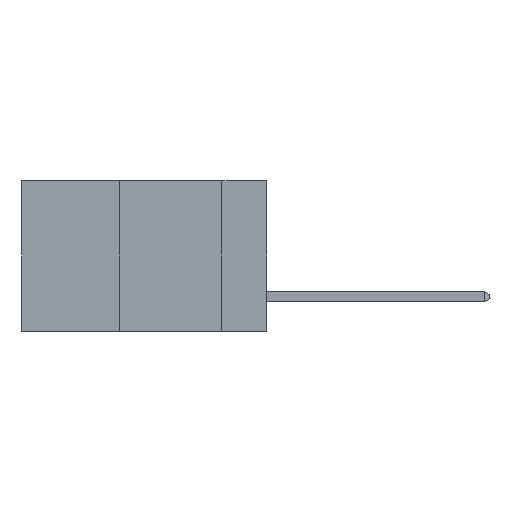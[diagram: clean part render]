
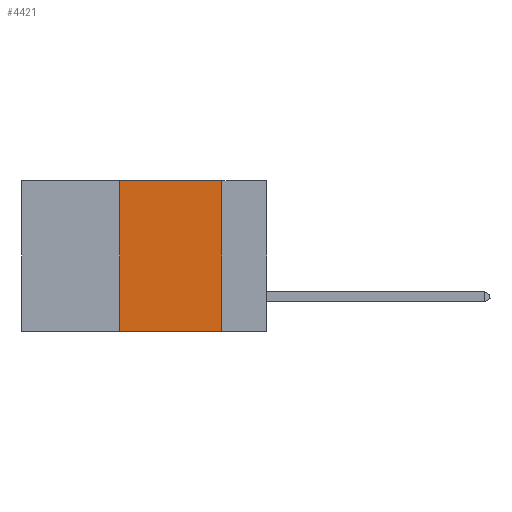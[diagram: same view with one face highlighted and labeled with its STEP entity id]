
A CAD part, left-side view. The second image highlights one B-rep face of the part: STEP entity #4421.
In plain terms, the highlighted planar face has unit normal (-1, 0, 0).
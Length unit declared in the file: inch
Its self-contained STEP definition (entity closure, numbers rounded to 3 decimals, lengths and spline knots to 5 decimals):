
#162 = DIRECTION ( 'NONE',  ( 1., 0., 0. ) ) ;
#515 = VECTOR ( 'NONE', #15361, 39.37008 ) ;
#859 = ORIENTED_EDGE ( 'NONE', *, *, #13508, .T. ) ;
#989 = FACE_OUTER_BOUND ( 'NONE', #6195, .T. ) ;
#1679 = CARTESIAN_POINT ( 'NONE',  ( 0., 0.6, -0.37 ) ) ;
#1713 = ORIENTED_EDGE ( 'NONE', *, *, #8844, .F. ) ;
#3783 = EDGE_CURVE ( 'NONE', #13636, #9212, #14231, .T. ) ;
#4421 = ADVANCED_FACE ( 'NONE', ( #989 ), #17350, .F. ) ;
#4846 = CARTESIAN_POINT ( 'NONE',  ( 0., 0.11, 0. ) ) ;
#4976 = LINE ( 'NONE', #8102, #515 ) ;
#6195 = EDGE_LOOP ( 'NONE', ( #6665, #7894, #1713, #859 ) ) ;
#6665 = ORIENTED_EDGE ( 'NONE', *, *, #19580, .F. ) ;
#7894 = ORIENTED_EDGE ( 'NONE', *, *, #3783, .F. ) ;
#8102 = CARTESIAN_POINT ( 'NONE',  ( 0., 0.36, 0. ) ) ;
#8215 = DIRECTION ( 'NONE',  ( 0., -1., 0. ) ) ;
#8844 = EDGE_CURVE ( 'NONE', #9439, #13636, #4976, .T. ) ;
#9212 = VERTEX_POINT ( 'NONE', #15399 ) ;
#9439 = VERTEX_POINT ( 'NONE', #16611 ) ;
#9733 = VECTOR ( 'NONE', #14005, 39.37008 ) ;
#12286 = CARTESIAN_POINT ( 'NONE',  ( 0., 0.6, 0. ) ) ;
#12391 = AXIS2_PLACEMENT_3D ( 'NONE', #15660, #162, #13972 ) ;
#13508 = EDGE_CURVE ( 'NONE', #9439, #14914, #20814, .T. ) ;
#13636 = VERTEX_POINT ( 'NONE', #19396 ) ;
#13972 = DIRECTION ( 'NONE',  ( 0., 0., -1. ) ) ;
#14005 = DIRECTION ( 'NONE',  ( 0., -1., 0. ) ) ;
#14231 = LINE ( 'NONE', #12286, #9733 ) ;
#14914 = VERTEX_POINT ( 'NONE', #17133 ) ;
#14917 = DIRECTION ( 'NONE',  ( 0., 0., -1. ) ) ;
#15268 = VECTOR ( 'NONE', #8215, 39.37008 ) ;
#15361 = DIRECTION ( 'NONE',  ( 0., 0., 1. ) ) ;
#15399 = CARTESIAN_POINT ( 'NONE',  ( 0., 0.11, 0. ) ) ;
#15660 = CARTESIAN_POINT ( 'NONE',  ( 0., 0.6, 0. ) ) ;
#16269 = LINE ( 'NONE', #4846, #18379 ) ;
#16611 = CARTESIAN_POINT ( 'NONE',  ( 0., 0.36, -0.37 ) ) ;
#17133 = CARTESIAN_POINT ( 'NONE',  ( 0., 0.11, -0.37 ) ) ;
#17350 = PLANE ( 'NONE',  #12391 ) ;
#18379 = VECTOR ( 'NONE', #14917, 39.37008 ) ;
#19396 = CARTESIAN_POINT ( 'NONE',  ( 0., 0.36, 0. ) ) ;
#19580 = EDGE_CURVE ( 'NONE', #9212, #14914, #16269, .T. ) ;
#20814 = LINE ( 'NONE', #1679, #15268 ) ;
